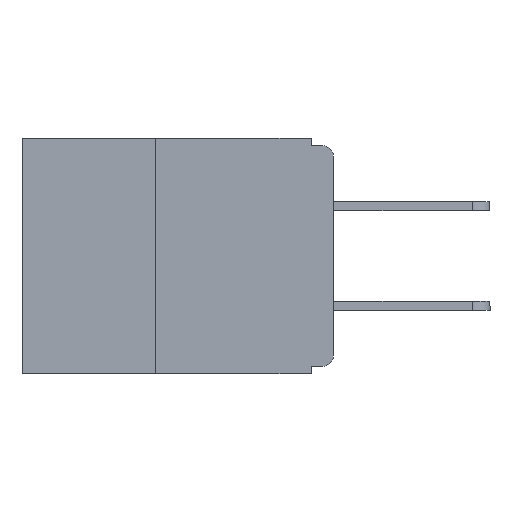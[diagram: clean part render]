
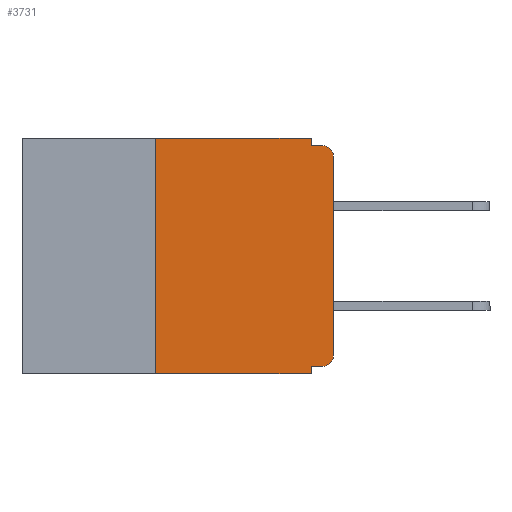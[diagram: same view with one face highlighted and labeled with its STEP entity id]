
A CAD part, left-side view. The second image highlights one B-rep face of the part: STEP entity #3731.
In plain terms, the highlighted planar face has unit normal (-1, 0, 0).
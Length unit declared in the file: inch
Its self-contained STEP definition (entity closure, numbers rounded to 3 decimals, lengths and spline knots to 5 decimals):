
#310 = DIRECTION ( 'NONE',  ( 0., 0., 1. ) ) ;
#658 = FACE_OUTER_BOUND ( 'NONE', #13934, .T. ) ;
#1086 = VERTEX_POINT ( 'NONE', #13601 ) ;
#2271 = AXIS2_PLACEMENT_3D ( 'NONE', #25705, #10536, #28152 ) ;
#3140 = EDGE_CURVE ( 'NONE', #15797, #21158, #24177, .T. ) ;
#3731 = ADVANCED_FACE ( 'NONE', ( #658 ), #20105, .F. ) ;
#3805 = ORIENTED_EDGE ( 'NONE', *, *, #5828, .F. ) ;
#3869 = LINE ( 'NONE', #5477, #9065 ) ;
#4984 = VERTEX_POINT ( 'NONE', #11055 ) ;
#5477 = CARTESIAN_POINT ( 'NONE',  ( 0., 0.031, 0. ) ) ;
#5599 = CIRCLE ( 'NONE', #19013, 0.015 ) ;
#5828 = EDGE_CURVE ( 'NONE', #9287, #16063, #27865, .T. ) ;
#6095 = ORIENTED_EDGE ( 'NONE', *, *, #27748, .T. ) ;
#6811 = CARTESIAN_POINT ( 'NONE',  ( 0., 0.437, -0.33 ) ) ;
#7060 = LINE ( 'NONE', #16269, #19853 ) ;
#8197 = VERTEX_POINT ( 'NONE', #26909 ) ;
#8680 = ORIENTED_EDGE ( 'NONE', *, *, #20821, .F. ) ;
#9065 = VECTOR ( 'NONE', #18353, 39.37008 ) ;
#9126 = EDGE_CURVE ( 'NONE', #4984, #1086, #28029, .T. ) ;
#9287 = VERTEX_POINT ( 'NONE', #28806 ) ;
#9321 = CARTESIAN_POINT ( 'NONE',  ( 0., 0., -0.01 ) ) ;
#9499 = ORIENTED_EDGE ( 'NONE', *, *, #28711, .F. ) ;
#9540 = VECTOR ( 'NONE', #9812, 39.37008 ) ;
#9812 = DIRECTION ( 'NONE',  ( 0., 0., 1. ) ) ;
#9842 = VERTEX_POINT ( 'NONE', #15761 ) ;
#10339 = CARTESIAN_POINT ( 'NONE',  ( 0., 0.015, -0.025 ) ) ;
#10478 = CARTESIAN_POINT ( 'NONE',  ( 0., 0.25, -0.33 ) ) ;
#10536 = DIRECTION ( 'NONE',  ( -1., 0., 0. ) ) ;
#11055 = CARTESIAN_POINT ( 'NONE',  ( 0., 0.015, -0.32 ) ) ;
#11058 = DIRECTION ( 'NONE',  ( 0., 1., 0. ) ) ;
#11450 = LINE ( 'NONE', #23647, #24084 ) ;
#12947 = DIRECTION ( 'NONE',  ( 0., 0., -1. ) ) ;
#13397 = VECTOR ( 'NONE', #26992, 39.37008 ) ;
#13601 = CARTESIAN_POINT ( 'NONE',  ( 0., 0., -0.305 ) ) ;
#13745 = VECTOR ( 'NONE', #310, 39.37008 ) ;
#13878 = CARTESIAN_POINT ( 'NONE',  ( 0., 0.031, -0.33 ) ) ;
#13934 = EDGE_LOOP ( 'NONE', ( #6095, #19318, #32196, #8680, #9499, #3805, #25958, #24485, #32312, #17132 ) ) ;
#14064 = EDGE_CURVE ( 'NONE', #9287, #21158, #26034, .T. ) ;
#14192 = LINE ( 'NONE', #9321, #13397 ) ;
#14322 = DIRECTION ( 'NONE',  ( 0., 0., -1. ) ) ;
#14976 = EDGE_CURVE ( 'NONE', #4984, #15797, #11450, .T. ) ;
#15761 = CARTESIAN_POINT ( 'NONE',  ( 0., 0.031, -0.01 ) ) ;
#15797 = VERTEX_POINT ( 'NONE', #19243 ) ;
#16063 = VERTEX_POINT ( 'NONE', #25484 ) ;
#16269 = CARTESIAN_POINT ( 'NONE',  ( 0., 0.437, 0. ) ) ;
#16363 = LINE ( 'NONE', #29807, #9540 ) ;
#17132 = ORIENTED_EDGE ( 'NONE', *, *, #9126, .T. ) ;
#17421 = EDGE_CURVE ( 'NONE', #24708, #18339, #5599, .T. ) ;
#18339 = VERTEX_POINT ( 'NONE', #31410 ) ;
#18353 = DIRECTION ( 'NONE',  ( 0., 0., -1. ) ) ;
#18794 = DIRECTION ( 'NONE',  ( 0., -1., 0. ) ) ;
#19013 = AXIS2_PLACEMENT_3D ( 'NONE', #10339, #27970, #12947 ) ;
#19093 = VECTOR ( 'NONE', #14322, 39.37008 ) ;
#19243 = CARTESIAN_POINT ( 'NONE',  ( 0., 0.031, -0.32 ) ) ;
#19318 = ORIENTED_EDGE ( 'NONE', *, *, #17421, .T. ) ;
#19522 = AXIS2_PLACEMENT_3D ( 'NONE', #20067, #20010, #20005 ) ;
#19853 = VECTOR ( 'NONE', #18794, 39.37008 ) ;
#20005 = DIRECTION ( 'NONE',  ( 0., 0., -1. ) ) ;
#20010 = DIRECTION ( 'NONE',  ( 1., 0., 0. ) ) ;
#20067 = CARTESIAN_POINT ( 'NONE',  ( 0., 0.437, 0. ) ) ;
#20105 = PLANE ( 'NONE',  #19522 ) ;
#20821 = EDGE_CURVE ( 'NONE', #8197, #9842, #3869, .T. ) ;
#21158 = VERTEX_POINT ( 'NONE', #27042 ) ;
#23647 = CARTESIAN_POINT ( 'NONE',  ( 0., 0., -0.32 ) ) ;
#24084 = VECTOR ( 'NONE', #11058, 39.37008 ) ;
#24177 = LINE ( 'NONE', #13878, #19093 ) ;
#24485 = ORIENTED_EDGE ( 'NONE', *, *, #3140, .F. ) ;
#24708 = VERTEX_POINT ( 'NONE', #30610 ) ;
#25484 = CARTESIAN_POINT ( 'NONE',  ( 0., 0.25, 0. ) ) ;
#25705 = CARTESIAN_POINT ( 'NONE',  ( 0., 0.015, -0.305 ) ) ;
#25958 = ORIENTED_EDGE ( 'NONE', *, *, #14064, .T. ) ;
#26034 = LINE ( 'NONE', #6811, #30981 ) ;
#26909 = CARTESIAN_POINT ( 'NONE',  ( 0., 0.031, 0. ) ) ;
#26992 = DIRECTION ( 'NONE',  ( 0., -1., 0. ) ) ;
#27042 = CARTESIAN_POINT ( 'NONE',  ( 0., 0.031, -0.33 ) ) ;
#27748 = EDGE_CURVE ( 'NONE', #1086, #24708, #16363, .T. ) ;
#27865 = LINE ( 'NONE', #10478, #13745 ) ;
#27970 = DIRECTION ( 'NONE',  ( -1., 0., 0. ) ) ;
#28029 = CIRCLE ( 'NONE', #2271, 0.015 ) ;
#28152 = DIRECTION ( 'NONE',  ( 0., 0., -1. ) ) ;
#28711 = EDGE_CURVE ( 'NONE', #16063, #8197, #7060, .T. ) ;
#28806 = CARTESIAN_POINT ( 'NONE',  ( 0., 0.25, -0.33 ) ) ;
#29543 = DIRECTION ( 'NONE',  ( 0., -1., 0. ) ) ;
#29807 = CARTESIAN_POINT ( 'NONE',  ( 0., 0., 0. ) ) ;
#30145 = EDGE_CURVE ( 'NONE', #9842, #18339, #14192, .T. ) ;
#30610 = CARTESIAN_POINT ( 'NONE',  ( 0., 0., -0.025 ) ) ;
#30981 = VECTOR ( 'NONE', #29543, 39.37008 ) ;
#31410 = CARTESIAN_POINT ( 'NONE',  ( 0., 0.015, -0.01 ) ) ;
#32196 = ORIENTED_EDGE ( 'NONE', *, *, #30145, .F. ) ;
#32312 = ORIENTED_EDGE ( 'NONE', *, *, #14976, .F. ) ;
